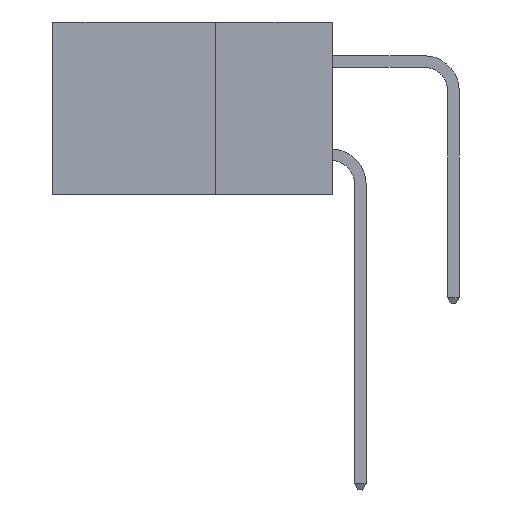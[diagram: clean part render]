
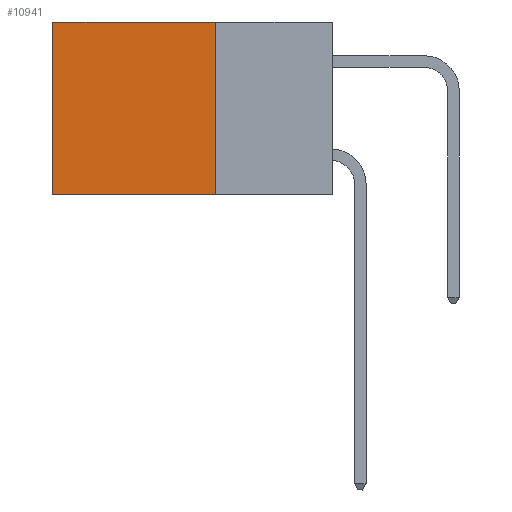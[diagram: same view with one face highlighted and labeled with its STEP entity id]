
A CAD part, left-side view. The second image highlights one B-rep face of the part: STEP entity #10941.
In plain terms, the highlighted planar face has unit normal (-1, 0, 0).
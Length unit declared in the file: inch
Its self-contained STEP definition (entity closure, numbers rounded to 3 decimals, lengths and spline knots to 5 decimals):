
#63 = FACE_OUTER_BOUND ( 'NONE', #24772, .T. ) ;
#665 = EDGE_CURVE ( 'NONE', #19221, #25304, #27958, .T. ) ;
#693 = CARTESIAN_POINT ( 'NONE',  ( 0.298, 0.25, 0. ) ) ;
#1488 = VERTEX_POINT ( 'NONE', #21119 ) ;
#2617 = AXIS2_PLACEMENT_3D ( 'NONE', #15645, #17850, #4652 ) ;
#3102 = VERTEX_POINT ( 'NONE', #693 ) ;
#3111 = CARTESIAN_POINT ( 'NONE',  ( 0.298, 0.6, 0. ) ) ;
#4571 = LINE ( 'NONE', #6288, #21464 ) ;
#4652 = DIRECTION ( 'NONE',  ( 0., 0., -1. ) ) ;
#5159 = CARTESIAN_POINT ( 'NONE',  ( 0.298, 0.25, -0.37 ) ) ;
#5391 = LINE ( 'NONE', #13684, #11928 ) ;
#6001 = ORIENTED_EDGE ( 'NONE', *, *, #9284, .T. ) ;
#6163 = ORIENTED_EDGE ( 'NONE', *, *, #13819, .T. ) ;
#6288 = CARTESIAN_POINT ( 'NONE',  ( 0.298, 0.25, 0. ) ) ;
#7983 = ORIENTED_EDGE ( 'NONE', *, *, #665, .F. ) ;
#9165 = CARTESIAN_POINT ( 'NONE',  ( 0.298, 0.25, -0.37 ) ) ;
#9284 = EDGE_CURVE ( 'NONE', #1488, #25304, #28003, .T. ) ;
#10357 = VECTOR ( 'NONE', #18453, 39.37008 ) ;
#10941 = ADVANCED_FACE ( 'NONE', ( #63 ), #13431, .F. ) ;
#11928 = VECTOR ( 'NONE', #15924, 39.37008 ) ;
#13431 = PLANE ( 'NONE',  #2617 ) ;
#13684 = CARTESIAN_POINT ( 'NONE',  ( 0.298, 0.25, 0. ) ) ;
#13819 = EDGE_CURVE ( 'NONE', #3102, #1488, #5391, .T. ) ;
#15645 = CARTESIAN_POINT ( 'NONE',  ( 0.298, 0.25, 0. ) ) ;
#15924 = DIRECTION ( 'NONE',  ( 0., 1., 0. ) ) ;
#16392 = DIRECTION ( 'NONE',  ( 0., 0., -1. ) ) ;
#17087 = EDGE_CURVE ( 'NONE', #3102, #19221, #4571, .T. ) ;
#17850 = DIRECTION ( 'NONE',  ( 1., 0., 0. ) ) ;
#18453 = DIRECTION ( 'NONE',  ( 0., 1., 0. ) ) ;
#19221 = VERTEX_POINT ( 'NONE', #9165 ) ;
#19331 = ORIENTED_EDGE ( 'NONE', *, *, #17087, .F. ) ;
#21119 = CARTESIAN_POINT ( 'NONE',  ( 0.298, 0.6, 0. ) ) ;
#21464 = VECTOR ( 'NONE', #26118, 39.37008 ) ;
#22233 = CARTESIAN_POINT ( 'NONE',  ( 0.298, 0.6, -0.37 ) ) ;
#22831 = VECTOR ( 'NONE', #16392, 39.37008 ) ;
#24772 = EDGE_LOOP ( 'NONE', ( #6001, #7983, #19331, #6163 ) ) ;
#25304 = VERTEX_POINT ( 'NONE', #22233 ) ;
#26118 = DIRECTION ( 'NONE',  ( 0., 0., -1. ) ) ;
#27958 = LINE ( 'NONE', #5159, #10357 ) ;
#28003 = LINE ( 'NONE', #3111, #22831 ) ;
